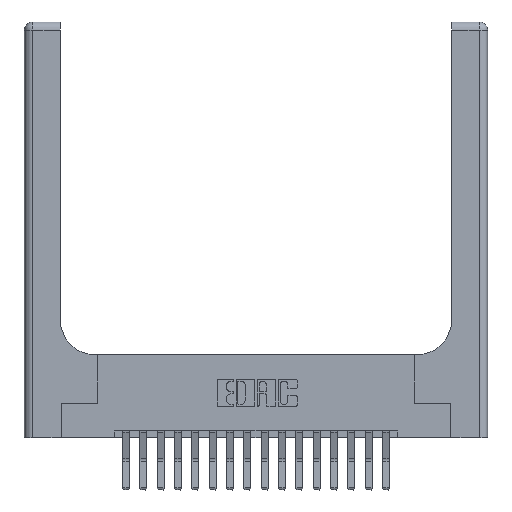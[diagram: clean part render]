
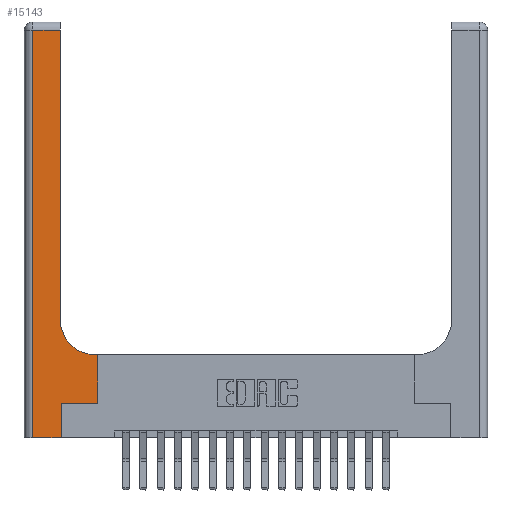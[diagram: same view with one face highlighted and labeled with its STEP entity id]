
A CAD part, top view. The second image highlights one B-rep face of the part: STEP entity #15143.
In plain terms, the highlighted planar face has unit normal (0, 0, 1).
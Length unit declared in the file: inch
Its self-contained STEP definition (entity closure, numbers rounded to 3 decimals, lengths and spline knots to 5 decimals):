
#596 = CARTESIAN_POINT ( 'NONE',  ( 0., 2.94, 0.37 ) ) ;
#1570 = VECTOR ( 'NONE', #15434, 39.37008 ) ;
#1598 = ORIENTED_EDGE ( 'NONE', *, *, #17070, .T. ) ;
#1736 = EDGE_CURVE ( 'NONE', #17907, #18614, #6300, .T. ) ;
#1795 = CARTESIAN_POINT ( 'NONE',  ( 0.528, 0.25, 0.37 ) ) ;
#2217 = DIRECTION ( 'NONE',  ( -1., 0., 0. ) ) ;
#2295 = VECTOR ( 'NONE', #14098, 39.37008 ) ;
#2666 = ORIENTED_EDGE ( 'NONE', *, *, #10132, .T. ) ;
#3807 = DIRECTION ( 'NONE',  ( 0., 0., -1. ) ) ;
#4003 = ORIENTED_EDGE ( 'NONE', *, *, #9848, .T. ) ;
#4167 = VECTOR ( 'NONE', #17349, 39.37008 ) ;
#4183 = EDGE_LOOP ( 'NONE', ( #2666, #1598, #10257, #9715, #4449, #5085, #14710, #4003, #12018 ) ) ;
#4406 = CARTESIAN_POINT ( 'NONE',  ( 0.26, 2.94, 0.37 ) ) ;
#4449 = ORIENTED_EDGE ( 'NONE', *, *, #14008, .T. ) ;
#4471 = CARTESIAN_POINT ( 'NONE',  ( 0.51, 0.6, 0.37 ) ) ;
#4783 = VECTOR ( 'NONE', #10597, 39.37008 ) ;
#5085 = ORIENTED_EDGE ( 'NONE', *, *, #9956, .T. ) ;
#5109 = VECTOR ( 'NONE', #6375, 39.37008 ) ;
#5114 = LINE ( 'NONE', #6516, #12408 ) ;
#5304 = PLANE ( 'NONE',  #9328 ) ;
#5512 = EDGE_CURVE ( 'NONE', #15679, #14293, #9764, .T. ) ;
#6056 = VERTEX_POINT ( 'NONE', #7136 ) ;
#6119 = VERTEX_POINT ( 'NONE', #11617 ) ;
#6300 = LINE ( 'NONE', #9398, #1570 ) ;
#6375 = DIRECTION ( 'NONE',  ( 0., 1., 0. ) ) ;
#6516 = CARTESIAN_POINT ( 'NONE',  ( 0.265, 0.25, 0.37 ) ) ;
#6613 = DIRECTION ( 'NONE',  ( -1., 0., 0. ) ) ;
#6781 = LINE ( 'NONE', #596, #8756 ) ;
#7136 = CARTESIAN_POINT ( 'NONE',  ( 0.528, 0.25, 0.37 ) ) ;
#7365 = CARTESIAN_POINT ( 'NONE',  ( 0.51, 0.85, 0.37 ) ) ;
#7459 = DIRECTION ( 'NONE',  ( 1., 0., 0. ) ) ;
#7912 = DIRECTION ( 'NONE',  ( 1., 0., 0. ) ) ;
#8016 = CARTESIAN_POINT ( 'NONE',  ( 0.26, 0.6, 0.37 ) ) ;
#8333 = LINE ( 'NONE', #15955, #4167 ) ;
#8756 = VECTOR ( 'NONE', #12749, 39.37008 ) ;
#9129 = AXIS2_PLACEMENT_3D ( 'NONE', #7365, #14894, #7459 ) ;
#9328 = AXIS2_PLACEMENT_3D ( 'NONE', #15833, #3807, #2217 ) ;
#9398 = CARTESIAN_POINT ( 'NONE',  ( 0., 0., 0.37 ) ) ;
#9715 = ORIENTED_EDGE ( 'NONE', *, *, #1736, .T. ) ;
#9719 = CARTESIAN_POINT ( 'NONE',  ( 0.528, 0.6, 0.37 ) ) ;
#9764 = CIRCLE ( 'NONE', #9129, 0.25 ) ;
#9800 = FACE_OUTER_BOUND ( 'NONE', #4183, .T. ) ;
#9848 = EDGE_CURVE ( 'NONE', #11746, #15679, #18651, .T. ) ;
#9956 = EDGE_CURVE ( 'NONE', #6119, #6056, #5114, .T. ) ;
#10132 = EDGE_CURVE ( 'NONE', #14293, #10153, #12093, .T. ) ;
#10153 = VERTEX_POINT ( 'NONE', #4406 ) ;
#10257 = ORIENTED_EDGE ( 'NONE', *, *, #13266, .T. ) ;
#10436 = CARTESIAN_POINT ( 'NONE',  ( 0.26, 0.85, 0.37 ) ) ;
#10597 = DIRECTION ( 'NONE',  ( 0., 1., 0. ) ) ;
#11121 = CARTESIAN_POINT ( 'NONE',  ( 0.06, 2.94, 0.37 ) ) ;
#11617 = CARTESIAN_POINT ( 'NONE',  ( 0.265, 0.25, 0.37 ) ) ;
#11746 = VERTEX_POINT ( 'NONE', #9719 ) ;
#12018 = ORIENTED_EDGE ( 'NONE', *, *, #5512, .T. ) ;
#12093 = LINE ( 'NONE', #16738, #4783 ) ;
#12310 = EDGE_CURVE ( 'NONE', #6056, #11746, #15406, .T. ) ;
#12408 = VECTOR ( 'NONE', #7912, 39.37008 ) ;
#12428 = CARTESIAN_POINT ( 'NONE',  ( 0.265, 0., 0.37 ) ) ;
#12749 = DIRECTION ( 'NONE',  ( -1., 0., 0. ) ) ;
#13266 = EDGE_CURVE ( 'NONE', #19064, #17907, #8333, .T. ) ;
#13977 = VECTOR ( 'NONE', #6613, 39.37008 ) ;
#14008 = EDGE_CURVE ( 'NONE', #18614, #6119, #16877, .T. ) ;
#14098 = DIRECTION ( 'NONE',  ( 0., 1., 0. ) ) ;
#14102 = CARTESIAN_POINT ( 'NONE',  ( 0.265, 0., 0.37 ) ) ;
#14293 = VERTEX_POINT ( 'NONE', #10436 ) ;
#14710 = ORIENTED_EDGE ( 'NONE', *, *, #12310, .T. ) ;
#14894 = DIRECTION ( 'NONE',  ( 0., 0., -1. ) ) ;
#15143 = ADVANCED_FACE ( 'NONE', ( #9800 ), #5304, .F. ) ;
#15406 = LINE ( 'NONE', #1795, #5109 ) ;
#15434 = DIRECTION ( 'NONE',  ( 1., 0., 0. ) ) ;
#15471 = CARTESIAN_POINT ( 'NONE',  ( 0.06, 0., 0.37 ) ) ;
#15679 = VERTEX_POINT ( 'NONE', #4471 ) ;
#15833 = CARTESIAN_POINT ( 'NONE',  ( 0., 3., 0.37 ) ) ;
#15955 = CARTESIAN_POINT ( 'NONE',  ( 0.06, 3., 0.37 ) ) ;
#16738 = CARTESIAN_POINT ( 'NONE',  ( 0.26, 3., 0.37 ) ) ;
#16877 = LINE ( 'NONE', #12428, #2295 ) ;
#17070 = EDGE_CURVE ( 'NONE', #10153, #19064, #6781, .T. ) ;
#17349 = DIRECTION ( 'NONE',  ( 0., -1., 0. ) ) ;
#17907 = VERTEX_POINT ( 'NONE', #15471 ) ;
#18614 = VERTEX_POINT ( 'NONE', #14102 ) ;
#18651 = LINE ( 'NONE', #8016, #13977 ) ;
#19064 = VERTEX_POINT ( 'NONE', #11121 ) ;
